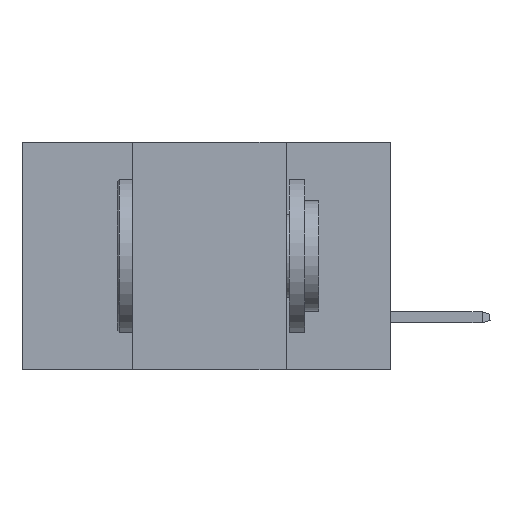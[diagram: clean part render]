
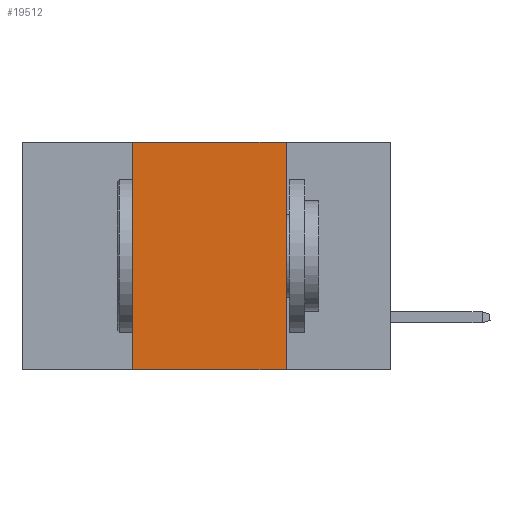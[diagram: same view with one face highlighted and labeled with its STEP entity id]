
A CAD part, left-side view. The second image highlights one B-rep face of the part: STEP entity #19512.
In plain terms, the highlighted planar face has unit normal (-1, 0, 0).
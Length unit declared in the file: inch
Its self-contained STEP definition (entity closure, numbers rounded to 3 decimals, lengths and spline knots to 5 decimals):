
#134 = VERTEX_POINT ( 'NONE', #3742 ) ;
#215 = CARTESIAN_POINT ( 'NONE',  ( 0., 0.6, 0. ) ) ;
#1858 = VECTOR ( 'NONE', #17479, 39.37008 ) ;
#2537 = CARTESIAN_POINT ( 'NONE',  ( 0., 0.17, -0.37 ) ) ;
#3665 = DIRECTION ( 'NONE',  ( 0., 0., 1. ) ) ;
#3742 = CARTESIAN_POINT ( 'NONE',  ( 0., 0.17, 0. ) ) ;
#3921 = CARTESIAN_POINT ( 'NONE',  ( 0., 0.42, 0. ) ) ;
#4018 = DIRECTION ( 'NONE',  ( 1., 0., 0. ) ) ;
#4469 = ORIENTED_EDGE ( 'NONE', *, *, #7414, .F. ) ;
#4872 = EDGE_CURVE ( 'NONE', #14363, #17124, #16594, .T. ) ;
#6134 = EDGE_CURVE ( 'NONE', #14363, #16558, #17673, .T. ) ;
#6714 = FACE_OUTER_BOUND ( 'NONE', #21747, .T. ) ;
#7414 = EDGE_CURVE ( 'NONE', #134, #17124, #19284, .T. ) ;
#7973 = VECTOR ( 'NONE', #19426, 39.37008 ) ;
#8564 = CARTESIAN_POINT ( 'NONE',  ( 0., 0.6, 0. ) ) ;
#9073 = VECTOR ( 'NONE', #20074, 39.37008 ) ;
#9208 = CARTESIAN_POINT ( 'NONE',  ( 0., 0.17, 0. ) ) ;
#10912 = EDGE_CURVE ( 'NONE', #16558, #134, #22436, .T. ) ;
#12658 = CARTESIAN_POINT ( 'NONE',  ( 0., 0.42, -0.37 ) ) ;
#14363 = VERTEX_POINT ( 'NONE', #12658 ) ;
#16558 = VERTEX_POINT ( 'NONE', #21100 ) ;
#16594 = LINE ( 'NONE', #22882, #1858 ) ;
#16814 = PLANE ( 'NONE',  #17117 ) ;
#16899 = DIRECTION ( 'NONE',  ( 0., 0., -1. ) ) ;
#17117 = AXIS2_PLACEMENT_3D ( 'NONE', #215, #4018, #16899 ) ;
#17124 = VERTEX_POINT ( 'NONE', #2537 ) ;
#17479 = DIRECTION ( 'NONE',  ( 0., -1., 0. ) ) ;
#17542 = ORIENTED_EDGE ( 'NONE', *, *, #6134, .F. ) ;
#17673 = LINE ( 'NONE', #3921, #21902 ) ;
#19087 = ORIENTED_EDGE ( 'NONE', *, *, #10912, .F. ) ;
#19284 = LINE ( 'NONE', #9208, #9073 ) ;
#19426 = DIRECTION ( 'NONE',  ( 0., -1., 0. ) ) ;
#19512 = ADVANCED_FACE ( 'NONE', ( #6714 ), #16814, .F. ) ;
#20074 = DIRECTION ( 'NONE',  ( 0., 0., -1. ) ) ;
#21100 = CARTESIAN_POINT ( 'NONE',  ( 0., 0.42, 0. ) ) ;
#21609 = ORIENTED_EDGE ( 'NONE', *, *, #4872, .T. ) ;
#21747 = EDGE_LOOP ( 'NONE', ( #4469, #19087, #17542, #21609 ) ) ;
#21902 = VECTOR ( 'NONE', #3665, 39.37008 ) ;
#22436 = LINE ( 'NONE', #8564, #7973 ) ;
#22882 = CARTESIAN_POINT ( 'NONE',  ( 0., 0.6, -0.37 ) ) ;
